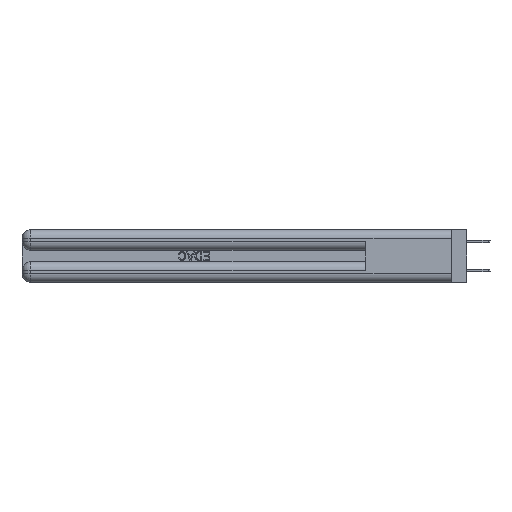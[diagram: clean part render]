
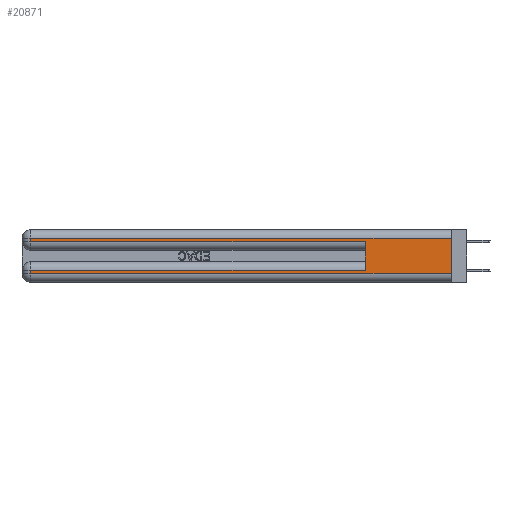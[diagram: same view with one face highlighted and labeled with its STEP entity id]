
A CAD part, left-side view. The second image highlights one B-rep face of the part: STEP entity #20871.
In plain terms, the highlighted planar face has unit normal (-1, 0, 0).
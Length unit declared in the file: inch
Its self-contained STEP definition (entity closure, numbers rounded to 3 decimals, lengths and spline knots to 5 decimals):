
#67 = EDGE_CURVE ( 'NONE', #26090, #2545, #12193, .T. ) ;
#590 = EDGE_CURVE ( 'NONE', #16441, #27575, #7367, .T. ) ;
#1771 = CARTESIAN_POINT ( 'NONE',  ( 0., 2.94, 0.31 ) ) ;
#2289 = DIRECTION ( 'NONE',  ( 0., -1., 0. ) ) ;
#2545 = VERTEX_POINT ( 'NONE', #28888 ) ;
#2650 = CARTESIAN_POINT ( 'NONE',  ( 0., 0., 0.06 ) ) ;
#4142 = ORIENTED_EDGE ( 'NONE', *, *, #21302, .T. ) ;
#4513 = CARTESIAN_POINT ( 'NONE',  ( 0., 0., 0.285 ) ) ;
#5047 = AXIS2_PLACEMENT_3D ( 'NONE', #18677, #12654, #33965 ) ;
#5677 = CARTESIAN_POINT ( 'NONE',  ( 0., 2.94, 0.37 ) ) ;
#5936 = ORIENTED_EDGE ( 'NONE', *, *, #18541, .T. ) ;
#6356 = CARTESIAN_POINT ( 'NONE',  ( 0., 2.94, 0.37 ) ) ;
#7305 = CARTESIAN_POINT ( 'NONE',  ( 0., 0.6, 0.145 ) ) ;
#7367 = LINE ( 'NONE', #22640, #38917 ) ;
#7977 = LINE ( 'NONE', #5677, #39514 ) ;
#8866 = VERTEX_POINT ( 'NONE', #9705 ) ;
#8938 = DIRECTION ( 'NONE',  ( 0., 0., 1. ) ) ;
#9705 = CARTESIAN_POINT ( 'NONE',  ( 0., 2.94, 0.285 ) ) ;
#9777 = EDGE_CURVE ( 'NONE', #37624, #27575, #34402, .T. ) ;
#9898 = CARTESIAN_POINT ( 'NONE',  ( 0., 2.94, 0.06 ) ) ;
#11045 = DIRECTION ( 'NONE',  ( 0., 0., -1. ) ) ;
#11752 = LINE ( 'NONE', #6356, #19885 ) ;
#12193 = LINE ( 'NONE', #7305, #34599 ) ;
#12654 = DIRECTION ( 'NONE',  ( 1., 0., 0. ) ) ;
#13642 = VECTOR ( 'NONE', #14896, 39.37008 ) ;
#14013 = ORIENTED_EDGE ( 'NONE', *, *, #34216, .T. ) ;
#14896 = DIRECTION ( 'NONE',  ( 0., 1., 0. ) ) ;
#16441 = VERTEX_POINT ( 'NONE', #32223 ) ;
#16696 = ORIENTED_EDGE ( 'NONE', *, *, #590, .F. ) ;
#17866 = DIRECTION ( 'NONE',  ( 0., 0., -1. ) ) ;
#18541 = EDGE_CURVE ( 'NONE', #8866, #2545, #26270, .T. ) ;
#18547 = PLANE ( 'NONE',  #5047 ) ;
#18677 = CARTESIAN_POINT ( 'NONE',  ( 0., 0., 0.37 ) ) ;
#19070 = VECTOR ( 'NONE', #29232, 39.37008 ) ;
#19785 = DIRECTION ( 'NONE',  ( 0., -1., 0. ) ) ;
#19885 = VECTOR ( 'NONE', #24648, 39.37008 ) ;
#20159 = ORIENTED_EDGE ( 'NONE', *, *, #28878, .T. ) ;
#20871 = ADVANCED_FACE ( 'NONE', ( #33215 ), #18547, .F. ) ;
#21263 = ORIENTED_EDGE ( 'NONE', *, *, #9777, .T. ) ;
#21302 = EDGE_CURVE ( 'NONE', #34704, #8866, #11752, .T. ) ;
#22640 = CARTESIAN_POINT ( 'NONE',  ( 0., 0., 0.37 ) ) ;
#24648 = DIRECTION ( 'NONE',  ( 0., 0., -1. ) ) ;
#26090 = VERTEX_POINT ( 'NONE', #33450 ) ;
#26172 = CARTESIAN_POINT ( 'NONE',  ( 0., 0., 0.31 ) ) ;
#26270 = LINE ( 'NONE', #4513, #33391 ) ;
#26307 = VECTOR ( 'NONE', #2289, 39.37008 ) ;
#26977 = LINE ( 'NONE', #30051, #13642 ) ;
#27575 = VERTEX_POINT ( 'NONE', #2650 ) ;
#28121 = LINE ( 'NONE', #26172, #19070 ) ;
#28176 = ORIENTED_EDGE ( 'NONE', *, *, #32181, .T. ) ;
#28878 = EDGE_CURVE ( 'NONE', #36557, #37624, #7977, .T. ) ;
#28888 = CARTESIAN_POINT ( 'NONE',  ( 0., 0.6, 0.285 ) ) ;
#29232 = DIRECTION ( 'NONE',  ( 0., 1., 0. ) ) ;
#30051 = CARTESIAN_POINT ( 'NONE',  ( 0., 0., 0.085 ) ) ;
#32181 = EDGE_CURVE ( 'NONE', #16441, #34704, #28121, .T. ) ;
#32223 = CARTESIAN_POINT ( 'NONE',  ( 0., 0., 0.31 ) ) ;
#32767 = CARTESIAN_POINT ( 'NONE',  ( 0., 0., 0.06 ) ) ;
#33215 = FACE_OUTER_BOUND ( 'NONE', #38615, .T. ) ;
#33391 = VECTOR ( 'NONE', #19785, 39.37008 ) ;
#33450 = CARTESIAN_POINT ( 'NONE',  ( 0., 0.6, 0.085 ) ) ;
#33965 = DIRECTION ( 'NONE',  ( 0., 0., -1. ) ) ;
#34216 = EDGE_CURVE ( 'NONE', #26090, #36557, #26977, .T. ) ;
#34402 = LINE ( 'NONE', #32767, #26307 ) ;
#34599 = VECTOR ( 'NONE', #8938, 39.37008 ) ;
#34704 = VERTEX_POINT ( 'NONE', #1771 ) ;
#35030 = CARTESIAN_POINT ( 'NONE',  ( 0., 2.94, 0.085 ) ) ;
#35965 = ORIENTED_EDGE ( 'NONE', *, *, #67, .F. ) ;
#36557 = VERTEX_POINT ( 'NONE', #35030 ) ;
#37624 = VERTEX_POINT ( 'NONE', #9898 ) ;
#38615 = EDGE_LOOP ( 'NONE', ( #16696, #28176, #4142, #5936, #35965, #14013, #20159, #21263 ) ) ;
#38917 = VECTOR ( 'NONE', #11045, 39.37008 ) ;
#39514 = VECTOR ( 'NONE', #17866, 39.37008 ) ;
